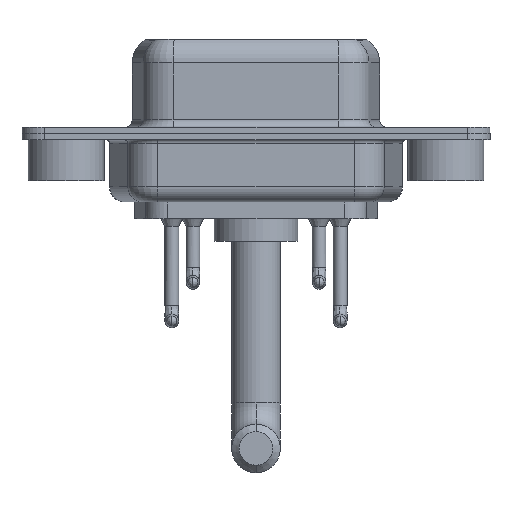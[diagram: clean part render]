
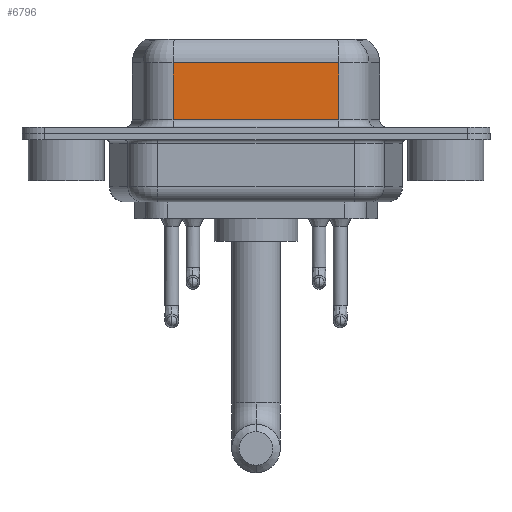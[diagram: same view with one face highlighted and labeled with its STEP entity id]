
A CAD part, front view. The second image highlights one B-rep face of the part: STEP entity #6796.
In plain terms, the highlighted planar face has unit normal (0, -1, 0).
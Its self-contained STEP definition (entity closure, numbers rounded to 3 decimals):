
#402 = EDGE_CURVE ( 'NONE', #11766, #4804, #8694, .T. ) ;
#628 = FACE_OUTER_BOUND ( 'NONE', #14494, .T. ) ;
#987 = VECTOR ( 'NONE', #12756, 1000. ) ;
#1462 = ORIENTED_EDGE ( 'NONE', *, *, #13296, .F. ) ;
#2297 = AXIS2_PLACEMENT_3D ( 'NONE', #8160, #5747, #15763 ) ;
#2436 = ORIENTED_EDGE ( 'NONE', *, *, #13594, .T. ) ;
#2565 = EDGE_CURVE ( 'NONE', #10588, #11706, #11251, .T. ) ;
#2650 = DIRECTION ( 'NONE',  ( 1., 0., 0. ) ) ;
#2682 = LINE ( 'NONE', #6538, #987 ) ;
#3612 = DIRECTION ( 'NONE',  ( 0., 0., -1. ) ) ;
#3831 = VECTOR ( 'NONE', #11352, 1000. ) ;
#4804 = VERTEX_POINT ( 'NONE', #11844 ) ;
#4845 = LINE ( 'NONE', #10064, #14694 ) ;
#5747 = DIRECTION ( 'NONE',  ( 0., 1., 0. ) ) ;
#6538 = CARTESIAN_POINT ( 'NONE',  ( 7.038, -3.95, 6.4 ) ) ;
#6796 = ADVANCED_FACE ( 'NONE', ( #628 ), #8074, .F. ) ;
#7112 = VECTOR ( 'NONE', #2650, 1000. ) ;
#7502 = CARTESIAN_POINT ( 'NONE',  ( 17.962, -3.95, 0.9 ) ) ;
#8074 = PLANE ( 'NONE',  #2297 ) ;
#8160 = CARTESIAN_POINT ( 'NONE',  ( 17.962, -3.95, 6.4 ) ) ;
#8694 = LINE ( 'NONE', #13959, #3831 ) ;
#10064 = CARTESIAN_POINT ( 'NONE',  ( 17.962, -3.95, 6.4 ) ) ;
#10588 = VERTEX_POINT ( 'NONE', #12283 ) ;
#11251 = LINE ( 'NONE', #7502, #7112 ) ;
#11352 = DIRECTION ( 'NONE',  ( -1., 0., 0. ) ) ;
#11580 = ORIENTED_EDGE ( 'NONE', *, *, #2565, .T. ) ;
#11706 = VERTEX_POINT ( 'NONE', #12716 ) ;
#11766 = VERTEX_POINT ( 'NONE', #15269 ) ;
#11844 = CARTESIAN_POINT ( 'NONE',  ( 7.038, -3.95, 4.65 ) ) ;
#12283 = CARTESIAN_POINT ( 'NONE',  ( 7.038, -3.95, 0.9 ) ) ;
#12303 = ORIENTED_EDGE ( 'NONE', *, *, #402, .T. ) ;
#12716 = CARTESIAN_POINT ( 'NONE',  ( 17.962, -3.95, 0.9 ) ) ;
#12756 = DIRECTION ( 'NONE',  ( 0., 0., -1. ) ) ;
#13296 = EDGE_CURVE ( 'NONE', #11766, #11706, #4845, .T. ) ;
#13594 = EDGE_CURVE ( 'NONE', #4804, #10588, #2682, .T. ) ;
#13959 = CARTESIAN_POINT ( 'NONE',  ( 17.962, -3.95, 4.65 ) ) ;
#14494 = EDGE_LOOP ( 'NONE', ( #1462, #12303, #2436, #11580 ) ) ;
#14694 = VECTOR ( 'NONE', #3612, 1000. ) ;
#15269 = CARTESIAN_POINT ( 'NONE',  ( 17.962, -3.95, 4.65 ) ) ;
#15763 = DIRECTION ( 'NONE',  ( -1., 0., 0. ) ) ;
